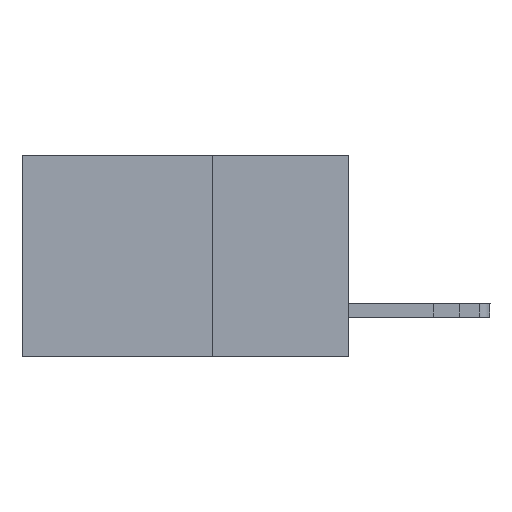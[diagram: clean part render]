
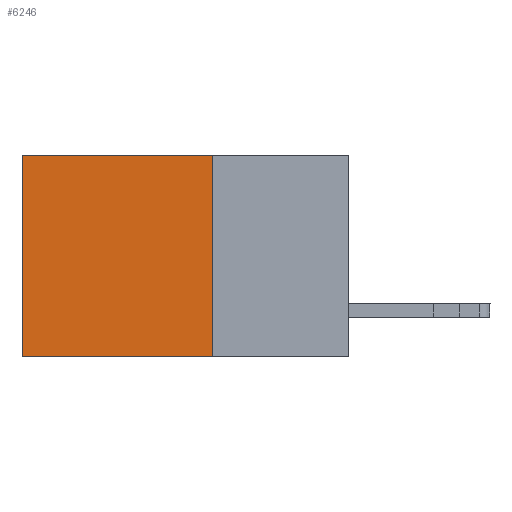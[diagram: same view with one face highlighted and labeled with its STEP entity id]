
A CAD part, left-side view. The second image highlights one B-rep face of the part: STEP entity #6246.
In plain terms, the highlighted planar face has unit normal (-1, 0, 0).
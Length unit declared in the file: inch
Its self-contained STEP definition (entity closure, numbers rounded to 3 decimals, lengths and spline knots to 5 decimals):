
#794 = DIRECTION ( 'NONE',  ( 0., 0., -1. ) ) ;
#1048 = VERTEX_POINT ( 'NONE', #5860 ) ;
#1155 = DIRECTION ( 'NONE',  ( 0., 1., 0. ) ) ;
#1371 = VERTEX_POINT ( 'NONE', #8537 ) ;
#1437 = CARTESIAN_POINT ( 'NONE',  ( 0.2615, 0.6, -0.37 ) ) ;
#1563 = LINE ( 'NONE', #6419, #10245 ) ;
#1573 = CARTESIAN_POINT ( 'NONE',  ( 0.2615, 0.25, -0.37 ) ) ;
#1977 = EDGE_CURVE ( 'NONE', #1371, #12099, #1563, .T. ) ;
#2415 = AXIS2_PLACEMENT_3D ( 'NONE', #6588, #5636, #10470 ) ;
#2454 = ORIENTED_EDGE ( 'NONE', *, *, #4493, .T. ) ;
#3606 = ORIENTED_EDGE ( 'NONE', *, *, #8510, .F. ) ;
#3825 = DIRECTION ( 'NONE',  ( 0., 0., -1. ) ) ;
#3933 = CARTESIAN_POINT ( 'NONE',  ( 0.2615, 0.25, 0. ) ) ;
#4493 = EDGE_CURVE ( 'NONE', #1048, #1371, #8761, .T. ) ;
#4739 = PLANE ( 'NONE',  #2415 ) ;
#5024 = CARTESIAN_POINT ( 'NONE',  ( 0.2615, 0.25, -0.37 ) ) ;
#5636 = DIRECTION ( 'NONE',  ( 1., 0., 0. ) ) ;
#5860 = CARTESIAN_POINT ( 'NONE',  ( 0.2615, 0.25, 0. ) ) ;
#5926 = VECTOR ( 'NONE', #3825, 39.37008 ) ;
#6246 = ADVANCED_FACE ( 'NONE', ( #9524 ), #4739, .F. ) ;
#6419 = CARTESIAN_POINT ( 'NONE',  ( 0.2615, 0.6, -0.37 ) ) ;
#6438 = VECTOR ( 'NONE', #1155, 39.37008 ) ;
#6588 = CARTESIAN_POINT ( 'NONE',  ( 0.2615, 0.25, -0.37 ) ) ;
#6750 = CARTESIAN_POINT ( 'NONE',  ( 0.2615, 0.25, -0.37 ) ) ;
#6877 = DIRECTION ( 'NONE',  ( 0., 1., 0. ) ) ;
#6964 = VERTEX_POINT ( 'NONE', #1573 ) ;
#7321 = ORIENTED_EDGE ( 'NONE', *, *, #12359, .F. ) ;
#7617 = EDGE_LOOP ( 'NONE', ( #10041, #7321, #3606, #2454 ) ) ;
#8510 = EDGE_CURVE ( 'NONE', #1048, #6964, #12548, .T. ) ;
#8537 = CARTESIAN_POINT ( 'NONE',  ( 0.2615, 0.6, 0. ) ) ;
#8761 = LINE ( 'NONE', #3933, #6438 ) ;
#9524 = FACE_OUTER_BOUND ( 'NONE', #7617, .T. ) ;
#9791 = LINE ( 'NONE', #5024, #10873 ) ;
#10041 = ORIENTED_EDGE ( 'NONE', *, *, #1977, .T. ) ;
#10245 = VECTOR ( 'NONE', #794, 39.37008 ) ;
#10470 = DIRECTION ( 'NONE',  ( 0., 0., -1. ) ) ;
#10873 = VECTOR ( 'NONE', #6877, 39.37008 ) ;
#12099 = VERTEX_POINT ( 'NONE', #1437 ) ;
#12359 = EDGE_CURVE ( 'NONE', #6964, #12099, #9791, .T. ) ;
#12548 = LINE ( 'NONE', #6750, #5926 ) ;
